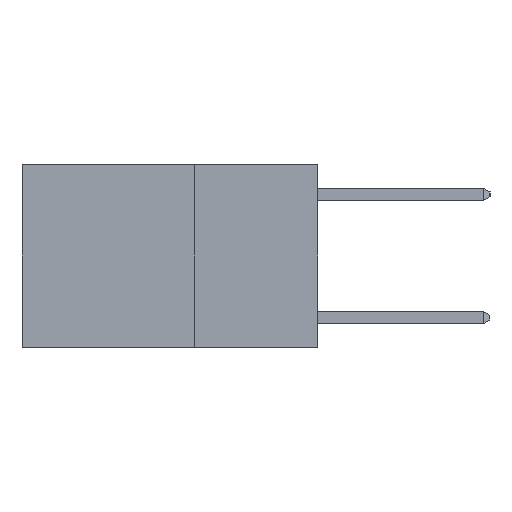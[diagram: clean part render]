
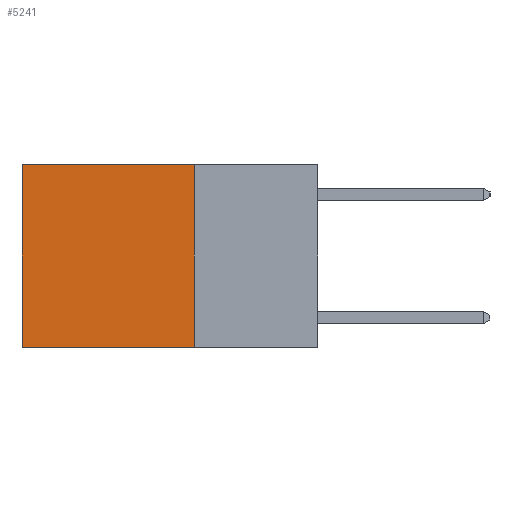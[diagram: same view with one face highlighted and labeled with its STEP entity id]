
A CAD part, left-side view. The second image highlights one B-rep face of the part: STEP entity #5241.
In plain terms, the highlighted planar face has unit normal (-1, 0, 0).
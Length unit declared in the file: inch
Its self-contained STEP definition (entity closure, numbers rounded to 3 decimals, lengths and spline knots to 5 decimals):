
#68 = AXIS2_PLACEMENT_3D ( 'NONE', #6875, #2580, #8505 ) ;
#541 = FACE_OUTER_BOUND ( 'NONE', #2129, .T. ) ;
#619 = EDGE_CURVE ( 'NONE', #2596, #5240, #1939, .T. ) ;
#683 = LINE ( 'NONE', #2048, #5371 ) ;
#980 = ORIENTED_EDGE ( 'NONE', *, *, #8061, .T. ) ;
#1100 = DIRECTION ( 'NONE',  ( 0., 0., -1. ) ) ;
#1137 = ORIENTED_EDGE ( 'NONE', *, *, #619, .F. ) ;
#1939 = LINE ( 'NONE', #8163, #8445 ) ;
#2048 = CARTESIAN_POINT ( 'NONE',  ( 0.2625, 0.6, 0. ) ) ;
#2129 = EDGE_LOOP ( 'NONE', ( #10450, #1137, #9464, #980 ) ) ;
#2248 = CARTESIAN_POINT ( 'NONE',  ( 0.2625, 0.25, 0. ) ) ;
#2580 = DIRECTION ( 'NONE',  ( 1., 0., 0. ) ) ;
#2596 = VERTEX_POINT ( 'NONE', #6181 ) ;
#3039 = LINE ( 'NONE', #7689, #7611 ) ;
#3307 = LINE ( 'NONE', #10430, #6692 ) ;
#3768 = CARTESIAN_POINT ( 'NONE',  ( 0.2625, 0.6, 0. ) ) ;
#5125 = DIRECTION ( 'NONE',  ( 0., 1., 0. ) ) ;
#5240 = VERTEX_POINT ( 'NONE', #6020 ) ;
#5241 = ADVANCED_FACE ( 'NONE', ( #541 ), #7710, .F. ) ;
#5371 = VECTOR ( 'NONE', #8004, 39.37008 ) ;
#5950 = EDGE_CURVE ( 'NONE', #8489, #2596, #3307, .T. ) ;
#5987 = EDGE_CURVE ( 'NONE', #10404, #5240, #683, .T. ) ;
#6020 = CARTESIAN_POINT ( 'NONE',  ( 0.2625, 0.6, -0.37 ) ) ;
#6181 = CARTESIAN_POINT ( 'NONE',  ( 0.2625, 0.25, -0.37 ) ) ;
#6692 = VECTOR ( 'NONE', #1100, 39.37008 ) ;
#6875 = CARTESIAN_POINT ( 'NONE',  ( 0.2625, 0.25, 0. ) ) ;
#7611 = VECTOR ( 'NONE', #5125, 39.37008 ) ;
#7689 = CARTESIAN_POINT ( 'NONE',  ( 0.2625, 0.25, 0. ) ) ;
#7710 = PLANE ( 'NONE',  #68 ) ;
#8004 = DIRECTION ( 'NONE',  ( 0., 0., -1. ) ) ;
#8061 = EDGE_CURVE ( 'NONE', #8489, #10404, #3039, .T. ) ;
#8163 = CARTESIAN_POINT ( 'NONE',  ( 0.2625, 0.25, -0.37 ) ) ;
#8445 = VECTOR ( 'NONE', #10631, 39.37008 ) ;
#8489 = VERTEX_POINT ( 'NONE', #2248 ) ;
#8505 = DIRECTION ( 'NONE',  ( 0., 0., -1. ) ) ;
#9464 = ORIENTED_EDGE ( 'NONE', *, *, #5950, .F. ) ;
#10404 = VERTEX_POINT ( 'NONE', #3768 ) ;
#10430 = CARTESIAN_POINT ( 'NONE',  ( 0.2625, 0.25, 0. ) ) ;
#10450 = ORIENTED_EDGE ( 'NONE', *, *, #5987, .T. ) ;
#10631 = DIRECTION ( 'NONE',  ( 0., 1., 0. ) ) ;
